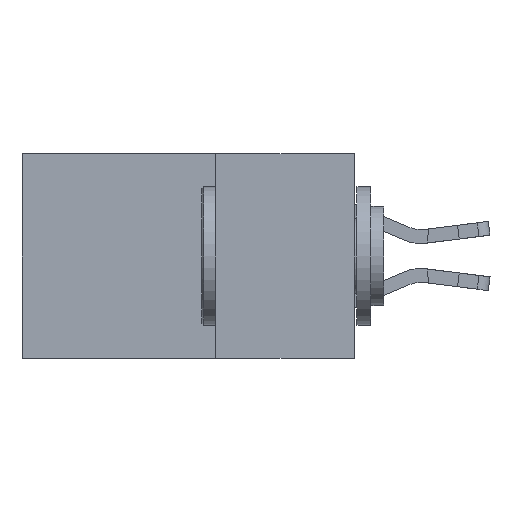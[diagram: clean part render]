
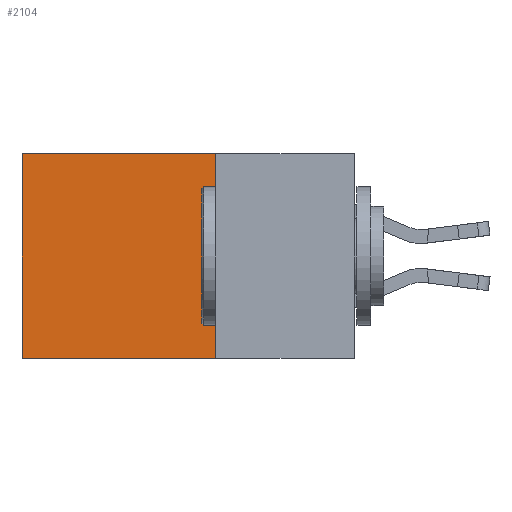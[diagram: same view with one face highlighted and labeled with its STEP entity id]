
A CAD part, left-side view. The second image highlights one B-rep face of the part: STEP entity #2104.
In plain terms, the highlighted planar face has unit normal (-1, 0, 0).
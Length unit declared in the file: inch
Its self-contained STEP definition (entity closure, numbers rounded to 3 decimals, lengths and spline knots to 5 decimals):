
#188 = ORIENTED_EDGE ( 'NONE', *, *, #12373, .T. ) ;
#240 = DIRECTION ( 'NONE',  ( 0., 1., 0. ) ) ;
#291 = CARTESIAN_POINT ( 'NONE',  ( 0.2615, 0.25, 0. ) ) ;
#366 = DIRECTION ( 'NONE',  ( 0., 1., 0. ) ) ;
#2104 = ADVANCED_FACE ( 'NONE', ( #9842 ), #10741, .F. ) ;
#2378 = VECTOR ( 'NONE', #366, 39.37008 ) ;
#2495 = CARTESIAN_POINT ( 'NONE',  ( 0.2615, 0.25, -0.37 ) ) ;
#3392 = DIRECTION ( 'NONE',  ( 1., 0., 0. ) ) ;
#3684 = ORIENTED_EDGE ( 'NONE', *, *, #8692, .T. ) ;
#3962 = VERTEX_POINT ( 'NONE', #291 ) ;
#4350 = ORIENTED_EDGE ( 'NONE', *, *, #9585, .F. ) ;
#4517 = AXIS2_PLACEMENT_3D ( 'NONE', #2495, #3392, #11461 ) ;
#4708 = CARTESIAN_POINT ( 'NONE',  ( 0.2615, 0.6, -0.37 ) ) ;
#5010 = VERTEX_POINT ( 'NONE', #4708 ) ;
#5291 = LINE ( 'NONE', #6163, #10419 ) ;
#5404 = EDGE_LOOP ( 'NONE', ( #3684, #10840, #4350, #188 ) ) ;
#6153 = CARTESIAN_POINT ( 'NONE',  ( 0.2615, 0.6, 0. ) ) ;
#6163 = CARTESIAN_POINT ( 'NONE',  ( 0.2615, 0.25, -0.37 ) ) ;
#6167 = EDGE_CURVE ( 'NONE', #11831, #5010, #5291, .T. ) ;
#6284 = CARTESIAN_POINT ( 'NONE',  ( 0.2615, 0.25, 0. ) ) ;
#7281 = DIRECTION ( 'NONE',  ( 0., 0., -1. ) ) ;
#7779 = VECTOR ( 'NONE', #7281, 39.37008 ) ;
#8088 = LINE ( 'NONE', #10162, #7779 ) ;
#8099 = CARTESIAN_POINT ( 'NONE',  ( 0.2615, 0.6, -0.37 ) ) ;
#8692 = EDGE_CURVE ( 'NONE', #8694, #5010, #10670, .T. ) ;
#8694 = VERTEX_POINT ( 'NONE', #6153 ) ;
#8808 = LINE ( 'NONE', #6284, #2378 ) ;
#9081 = DIRECTION ( 'NONE',  ( 0., 0., -1. ) ) ;
#9585 = EDGE_CURVE ( 'NONE', #3962, #11831, #8088, .T. ) ;
#9813 = CARTESIAN_POINT ( 'NONE',  ( 0.2615, 0.25, -0.37 ) ) ;
#9842 = FACE_OUTER_BOUND ( 'NONE', #5404, .T. ) ;
#10162 = CARTESIAN_POINT ( 'NONE',  ( 0.2615, 0.25, -0.37 ) ) ;
#10374 = VECTOR ( 'NONE', #9081, 39.37008 ) ;
#10419 = VECTOR ( 'NONE', #240, 39.37008 ) ;
#10670 = LINE ( 'NONE', #8099, #10374 ) ;
#10741 = PLANE ( 'NONE',  #4517 ) ;
#10840 = ORIENTED_EDGE ( 'NONE', *, *, #6167, .F. ) ;
#11461 = DIRECTION ( 'NONE',  ( 0., 0., -1. ) ) ;
#11831 = VERTEX_POINT ( 'NONE', #9813 ) ;
#12373 = EDGE_CURVE ( 'NONE', #3962, #8694, #8808, .T. ) ;
